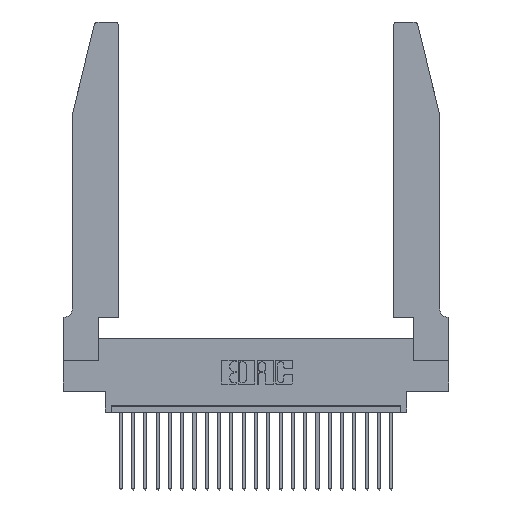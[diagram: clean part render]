
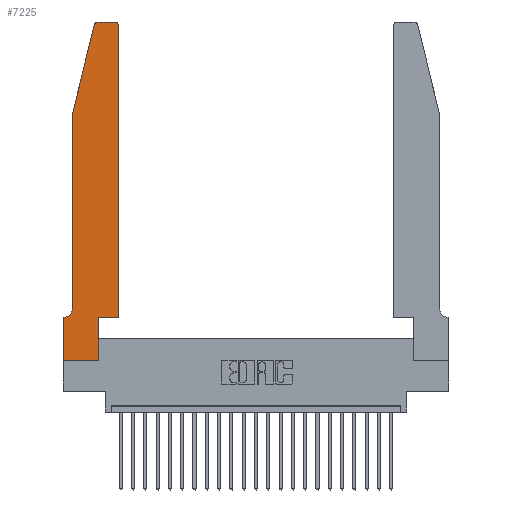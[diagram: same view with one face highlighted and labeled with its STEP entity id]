
A CAD part, top view. The second image highlights one B-rep face of the part: STEP entity #7225.
In plain terms, the highlighted planar face has unit normal (0, 0, 1).
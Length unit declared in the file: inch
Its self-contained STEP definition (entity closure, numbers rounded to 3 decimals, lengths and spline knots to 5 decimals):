
#549 = LINE ( 'NONE', #20161, #5379 ) ;
#552 = DIRECTION ( 'NONE',  ( 1., 0., 0. ) ) ;
#699 = VERTEX_POINT ( 'NONE', #4694 ) ;
#773 = CARTESIAN_POINT ( 'NONE',  ( 0.4505, 0.35, 0.37 ) ) ;
#923 = CARTESIAN_POINT ( 'NONE',  ( 0.0055, 0.35, 0.37 ) ) ;
#988 = CARTESIAN_POINT ( 'NONE',  ( 0.2865, 0.35, 0.37 ) ) ;
#1096 = DIRECTION ( 'NONE',  ( -1., 0., 0. ) ) ;
#1318 = EDGE_CURVE ( 'NONE', #6565, #2565, #9992, .T. ) ;
#1495 = LINE ( 'NONE', #17158, #6618 ) ;
#1679 = ORIENTED_EDGE ( 'NONE', *, *, #10362, .T. ) ;
#1704 = ORIENTED_EDGE ( 'NONE', *, *, #14973, .T. ) ;
#2055 = LINE ( 'NONE', #988, #13693 ) ;
#2565 = VERTEX_POINT ( 'NONE', #923 ) ;
#3116 = LINE ( 'NONE', #18477, #12040 ) ;
#3224 = CARTESIAN_POINT ( 'NONE',  ( 0.2605, 2.75, 0.37 ) ) ;
#3397 = VERTEX_POINT ( 'NONE', #20794 ) ;
#3533 = CARTESIAN_POINT ( 'NONE',  ( 0., 0.35, 0.37 ) ) ;
#3910 = VECTOR ( 'NONE', #1096, 39.37008 ) ;
#4006 = LINE ( 'NONE', #6868, #10238 ) ;
#4290 = CARTESIAN_POINT ( 'NONE',  ( 0.0755, 2., 0.37 ) ) ;
#4673 = VERTEX_POINT ( 'NONE', #21029 ) ;
#4694 = CARTESIAN_POINT ( 'NONE',  ( 0.0755, 2., 0.37 ) ) ;
#5294 = DIRECTION ( 'NONE',  ( 1., 0., 0. ) ) ;
#5379 = VECTOR ( 'NONE', #12664, 39.37008 ) ;
#5941 = CARTESIAN_POINT ( 'NONE',  ( 0.284, 2.75, 0.37 ) ) ;
#6458 = ORIENTED_EDGE ( 'NONE', *, *, #20686, .T. ) ;
#6565 = VERTEX_POINT ( 'NONE', #24491 ) ;
#6618 = VECTOR ( 'NONE', #20705, 39.37008 ) ;
#6868 = CARTESIAN_POINT ( 'NONE',  ( 0.4505, 0.35, 0.37 ) ) ;
#7225 = ADVANCED_FACE ( 'NONE', ( #15639 ), #9291, .T. ) ;
#7261 = EDGE_LOOP ( 'NONE', ( #1704, #21794, #16731, #23673, #16641, #14269, #20046, #6458, #17232, #23923, #12541, #1679 ) ) ;
#8925 = DIRECTION ( 'NONE',  ( -0.239, -0.971, 0. ) ) ;
#9156 = VERTEX_POINT ( 'NONE', #5941 ) ;
#9291 = PLANE ( 'NONE',  #14012 ) ;
#9442 = EDGE_CURVE ( 'NONE', #12130, #3397, #549, .T. ) ;
#9536 = CARTESIAN_POINT ( 'NONE',  ( 0., 0., 0.37 ) ) ;
#9664 = AXIS2_PLACEMENT_3D ( 'NONE', #15973, #12010, #552 ) ;
#9825 = VERTEX_POINT ( 'NONE', #23436 ) ;
#9931 = CARTESIAN_POINT ( 'NONE',  ( 0.0055, 0.42, 0.37 ) ) ;
#9992 = CIRCLE ( 'NONE', #10772, 0.07 ) ;
#10238 = VECTOR ( 'NONE', #10652, 39.37008 ) ;
#10362 = EDGE_CURVE ( 'NONE', #3397, #9825, #14004, .T. ) ;
#10652 = DIRECTION ( 'NONE',  ( 1., 0., 0. ) ) ;
#10685 = EDGE_CURVE ( 'NONE', #24470, #13419, #2055, .T. ) ;
#10772 = AXIS2_PLACEMENT_3D ( 'NONE', #9931, #23534, #19515 ) ;
#10859 = VERTEX_POINT ( 'NONE', #16976 ) ;
#11046 = CIRCLE ( 'NONE', #9664, 0.03 ) ;
#11584 = VECTOR ( 'NONE', #15816, 39.37008 ) ;
#12010 = DIRECTION ( 'NONE',  ( 0., 0., 1. ) ) ;
#12040 = VECTOR ( 'NONE', #8925, 39.37008 ) ;
#12126 = AXIS2_PLACEMENT_3D ( 'NONE', #18298, #20206, #23840 ) ;
#12130 = VERTEX_POINT ( 'NONE', #773 ) ;
#12171 = VECTOR ( 'NONE', #13764, 39.37008 ) ;
#12541 = ORIENTED_EDGE ( 'NONE', *, *, #9442, .T. ) ;
#12664 = DIRECTION ( 'NONE',  ( 0., 1., 0. ) ) ;
#13025 = DIRECTION ( 'NONE',  ( 0., 0., 1. ) ) ;
#13058 = VECTOR ( 'NONE', #21361, 39.37008 ) ;
#13419 = VERTEX_POINT ( 'NONE', #18324 ) ;
#13693 = VECTOR ( 'NONE', #16325, 39.37008 ) ;
#13764 = DIRECTION ( 'NONE',  ( 0., -1., 0. ) ) ;
#14004 = CIRCLE ( 'NONE', #12126, 0.03 ) ;
#14012 = AXIS2_PLACEMENT_3D ( 'NONE', #3533, #13025, #5294 ) ;
#14269 = ORIENTED_EDGE ( 'NONE', *, *, #22543, .T. ) ;
#14973 = EDGE_CURVE ( 'NONE', #9825, #9156, #19774, .T. ) ;
#15357 = EDGE_CURVE ( 'NONE', #9156, #4673, #11046, .T. ) ;
#15639 = FACE_OUTER_BOUND ( 'NONE', #7261, .T. ) ;
#15767 = EDGE_CURVE ( 'NONE', #10859, #16831, #19713, .T. ) ;
#15816 = DIRECTION ( 'NONE',  ( 0., -1., 0. ) ) ;
#15887 = CARTESIAN_POINT ( 'NONE',  ( 0.0755, 0.35, 0.37 ) ) ;
#15973 = CARTESIAN_POINT ( 'NONE',  ( 0.284, 2.72, 0.37 ) ) ;
#16325 = DIRECTION ( 'NONE',  ( 0., 1., 0. ) ) ;
#16641 = ORIENTED_EDGE ( 'NONE', *, *, #1318, .T. ) ;
#16717 = LINE ( 'NONE', #4290, #11584 ) ;
#16731 = ORIENTED_EDGE ( 'NONE', *, *, #19298, .T. ) ;
#16831 = VERTEX_POINT ( 'NONE', #21412 ) ;
#16976 = CARTESIAN_POINT ( 'NONE',  ( 0., 0.35, 0.37 ) ) ;
#17158 = CARTESIAN_POINT ( 'NONE',  ( 0., 0., 0.37 ) ) ;
#17232 = ORIENTED_EDGE ( 'NONE', *, *, #10685, .T. ) ;
#17872 = LINE ( 'NONE', #15887, #13058 ) ;
#18298 = CARTESIAN_POINT ( 'NONE',  ( 0.4205, 2.72, 0.37 ) ) ;
#18324 = CARTESIAN_POINT ( 'NONE',  ( 0.2865, 0.35, 0.37 ) ) ;
#18477 = CARTESIAN_POINT ( 'NONE',  ( 0.0755, 2., 0.37 ) ) ;
#19298 = EDGE_CURVE ( 'NONE', #4673, #699, #3116, .T. ) ;
#19305 = EDGE_CURVE ( 'NONE', #13419, #12130, #4006, .T. ) ;
#19515 = DIRECTION ( 'NONE',  ( -1., 0., 0. ) ) ;
#19713 = LINE ( 'NONE', #9536, #12171 ) ;
#19774 = LINE ( 'NONE', #3224, #3910 ) ;
#20046 = ORIENTED_EDGE ( 'NONE', *, *, #15767, .T. ) ;
#20161 = CARTESIAN_POINT ( 'NONE',  ( 0.4505, 0.35, 0.37 ) ) ;
#20206 = DIRECTION ( 'NONE',  ( 0., 0., 1. ) ) ;
#20686 = EDGE_CURVE ( 'NONE', #16831, #24470, #1495, .T. ) ;
#20705 = DIRECTION ( 'NONE',  ( 1., 0., 0. ) ) ;
#20794 = CARTESIAN_POINT ( 'NONE',  ( 0.4505, 2.72, 0.37 ) ) ;
#21029 = CARTESIAN_POINT ( 'NONE',  ( 0.25487, 2.72718, 0.37 ) ) ;
#21361 = DIRECTION ( 'NONE',  ( -1., 0., 0. ) ) ;
#21412 = CARTESIAN_POINT ( 'NONE',  ( 0., 0., 0.37 ) ) ;
#21794 = ORIENTED_EDGE ( 'NONE', *, *, #15357, .T. ) ;
#22051 = EDGE_CURVE ( 'NONE', #699, #6565, #16717, .T. ) ;
#22543 = EDGE_CURVE ( 'NONE', #2565, #10859, #17872, .T. ) ;
#22767 = CARTESIAN_POINT ( 'NONE',  ( 0.2865, 0., 0.37 ) ) ;
#23436 = CARTESIAN_POINT ( 'NONE',  ( 0.4205, 2.75, 0.37 ) ) ;
#23534 = DIRECTION ( 'NONE',  ( 0., 0., -1. ) ) ;
#23673 = ORIENTED_EDGE ( 'NONE', *, *, #22051, .T. ) ;
#23840 = DIRECTION ( 'NONE',  ( 1., 0., 0. ) ) ;
#23923 = ORIENTED_EDGE ( 'NONE', *, *, #19305, .T. ) ;
#24470 = VERTEX_POINT ( 'NONE', #22767 ) ;
#24491 = CARTESIAN_POINT ( 'NONE',  ( 0.0755, 0.42, 0.37 ) ) ;
